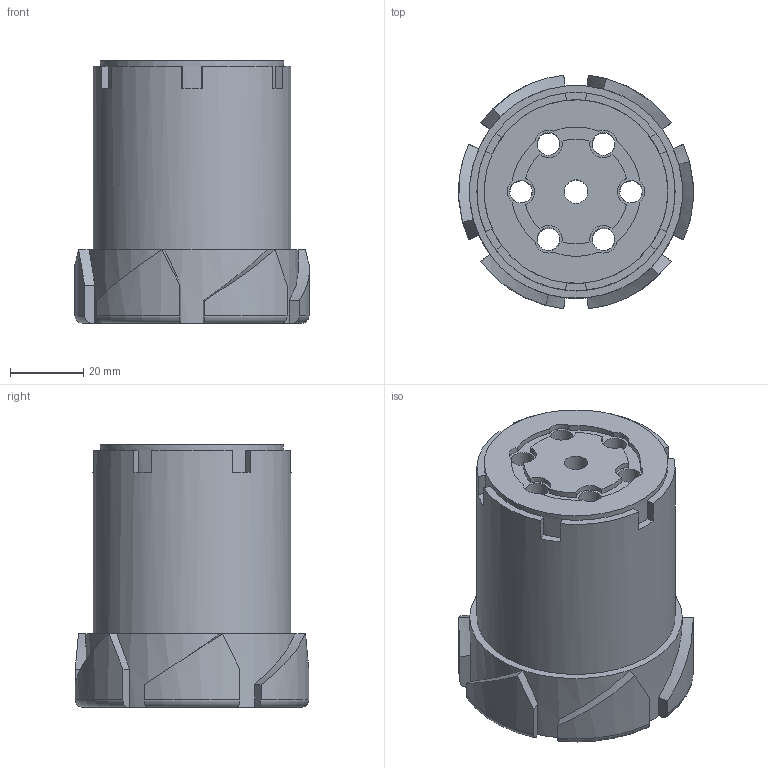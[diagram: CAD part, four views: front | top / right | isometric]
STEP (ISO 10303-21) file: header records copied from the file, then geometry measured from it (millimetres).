
FILE_DESCRIPTION((''),'2;1');
FILE_NAME('PM522NYLONFrontCylinderAssy2.stp','2015-10-01T18:19:03',('JamesRPatrick'),(''),'Autodesk Inventor 2012','Autodesk Inventor 2012','');
FILE_SCHEMA(('AUTOMOTIVE_DESIGN { 1 0 10303 214 1 1 1 1 }'));
Length unit declared in the file: millimetre
Products named in the file (3): PM522NYLONFrontCylinderAssy2.iam (LevelofDetail1); PM522NYLONFrontIndexRing2; PM522NYLONCylinder2
Assembly tree (2 placements, depth 2):
  PM522NYLONFrontCylinderAssy2.iam (LevelofDetail1)
    PM522NYLONFrontIndexRing2
    PM522NYLONCylinder2
Bounding box: 63.89 x 63.65 x 71.5 mm (x, y, z)
Volume: 160026.4 mm3; surface area: 35907.1 mm2
Topology: 2 solids, 2 shells, 190 faces, 547 edges, 363 vertices
Faces by surface type: plane 78, bspline 60, cylinder 46, torus 6
Full cylindrical faces by diameter (mm): 6.2 x6, 6.4 x1, 50 x1, 54 x2
Entity records: 8138 total; most frequent: CARTESIAN_POINT 3459, ORIENTED_EDGE 1044, DIRECTION 864, EDGE_CURVE 522, AXIS2_PLACEMENT_3D 375, VERTEX_POINT 348, CIRCLE 240, EDGE_LOOP 218
